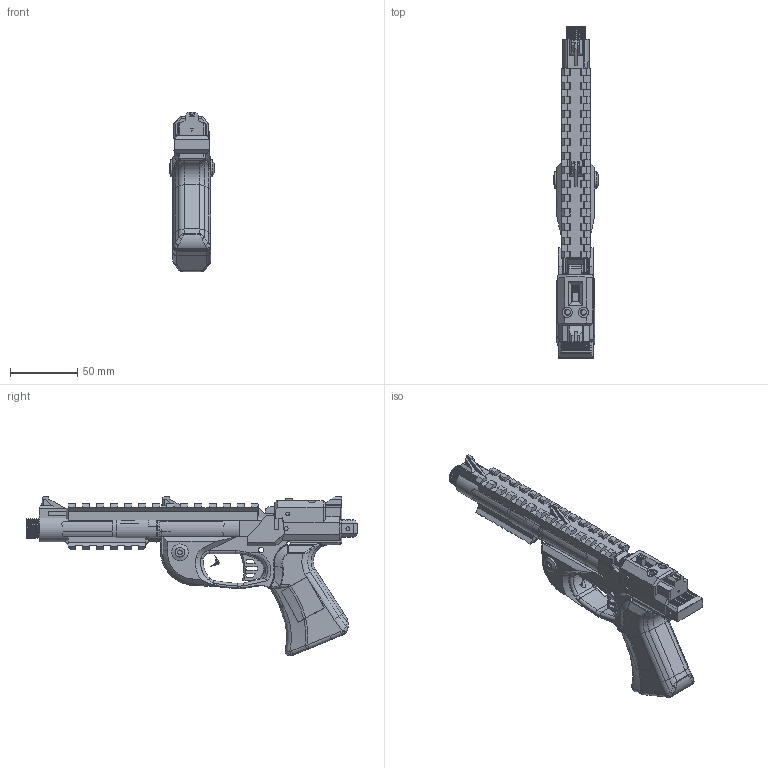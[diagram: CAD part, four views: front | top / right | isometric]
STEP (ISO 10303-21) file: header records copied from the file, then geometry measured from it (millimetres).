
FILE_DESCRIPTION(/* description */ (''),/* implementation_level */ '2;1');
FILE_NAME(/* name */ 'COVID-22 V.3 v3.step',/* time_stamp */ '2023-02-23T09:51:29-06:00',/* author */ (''),/* organization */ (''),/* preprocessor_version */ 'ST-DEVELOPER v19.2',/* originating_system */ 'Autodesk Translation Framework v11.17.0.187',/* authorisation */ '');
FILE_SCHEMA (('AUTOMOTIVE_DESIGN { 1 0 10303 214 3 1 1 }'));
Products named in the file (8): COVID-22 V.3; FGC; striker; Trigger; Barrels; BarrelCatchParts; Frame+Parts; MuzzleDevices
Assembly tree (7 placements, depth 3):
  COVID-22 V.3
    FGC
      striker
      Trigger
    Barrels
    BarrelCatchParts
    Frame+Parts
    MuzzleDevices
Bounding box: 33.65 x 247.06 x 118.59 mm (x, y, z)
Volume: 330808.5 mm3; surface area: 132352.1 mm2
Topology: 19 solids, 19 shells, 2220 faces, 6484 edges, 4324 vertices
Faces by surface type: plane 1242, bspline 474, cylinder 382, cone 72, torus 47, sphere 3
Full cylindrical faces by diameter (mm): 1 x1, 2.793 x8, 3 x2, 3.2 x1, 3.5 x2, 3.969 x1, 4 x2, 4.15 x2, 4.21 x1, 4.4 x2, 7 x1, 7.979 x1, 8 x6, 8.012 x3, 8.14 x5, 8.205 x6, 8.866 x1, 8.9 x1, 9.445 x6, 9.64 x3, 11.618 x10, 12.5 x2, 12.619 x10, 13.137 x12, 13.8 x6, 14.4 x12, 15.203 x6, 20 x1, 20.2 x1
Entity records: 144683 total; most frequent: CARTESIAN_POINT 89286, ORIENTED_EDGE 12916, DIRECTION 9265, EDGE_CURVE 6458, VERTEX_POINT 4322, LINE 3901, VECTOR 3901, AXIS2_PLACEMENT_3D 2682
